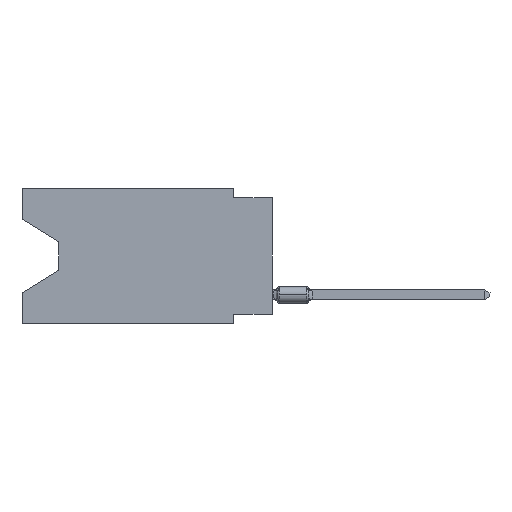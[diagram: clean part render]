
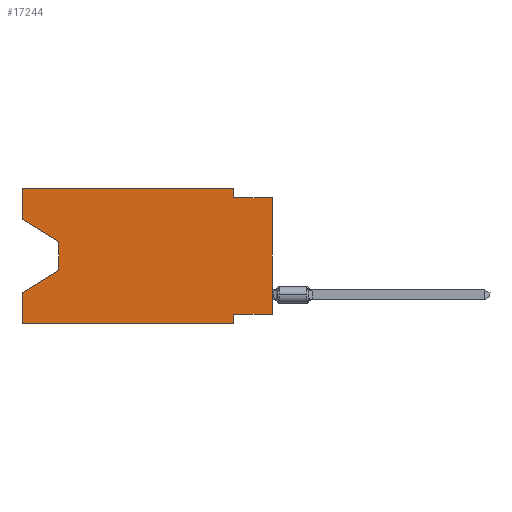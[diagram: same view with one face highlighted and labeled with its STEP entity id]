
A CAD part, left-side view. The second image highlights one B-rep face of the part: STEP entity #17244.
In plain terms, the highlighted planar face has unit normal (-1, 0, 0).
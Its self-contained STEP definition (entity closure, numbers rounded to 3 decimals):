
#54 = VECTOR ( 'NONE', #8513, 1000. ) ;
#129 = VERTEX_POINT ( 'NONE', #4464 ) ;
#520 = DIRECTION ( 'NONE',  ( 0., 0., 1. ) ) ;
#578 = CARTESIAN_POINT ( 'NONE',  ( 0., 2.54, 0. ) ) ;
#824 = CARTESIAN_POINT ( 'NONE',  ( 0., 2.54, -8.89 ) ) ;
#1201 = ORIENTED_EDGE ( 'NONE', *, *, #9714, .F. ) ;
#1211 = CARTESIAN_POINT ( 'NONE',  ( 0., 13.97, -5.385 ) ) ;
#1438 = CARTESIAN_POINT ( 'NONE',  ( 0., 16.383, -8.89 ) ) ;
#1601 = VECTOR ( 'NONE', #7014, 1000. ) ;
#1841 = EDGE_CURVE ( 'NONE', #129, #2615, #18291, .T. ) ;
#1871 = VECTOR ( 'NONE', #10089, 1000. ) ;
#1890 = VECTOR ( 'NONE', #2904, 1000. ) ;
#1977 = CARTESIAN_POINT ( 'NONE',  ( 0., 16.383, 0. ) ) ;
#2011 = LINE ( 'NONE', #16816, #14824 ) ;
#2221 = ORIENTED_EDGE ( 'NONE', *, *, #5392, .F. ) ;
#2327 = LINE ( 'NONE', #15957, #54 ) ;
#2352 = LINE ( 'NONE', #11203, #17663 ) ;
#2615 = VERTEX_POINT ( 'NONE', #17131 ) ;
#2904 = DIRECTION ( 'NONE',  ( 0., 0., -1. ) ) ;
#2983 = EDGE_CURVE ( 'NONE', #18612, #15103, #2011, .T. ) ;
#3115 = DIRECTION ( 'NONE',  ( 0., -1., 0. ) ) ;
#3797 = CARTESIAN_POINT ( 'NONE',  ( 0., 16.383, -6.852 ) ) ;
#3887 = EDGE_CURVE ( 'NONE', #11784, #18872, #2352, .T. ) ;
#3984 = CARTESIAN_POINT ( 'NONE',  ( 0., 16.383, -8.89 ) ) ;
#4029 = VECTOR ( 'NONE', #14144, 1000. ) ;
#4115 = CARTESIAN_POINT ( 'NONE',  ( 0., 0., -8.255 ) ) ;
#4148 = ORIENTED_EDGE ( 'NONE', *, *, #18192, .T. ) ;
#4203 = ORIENTED_EDGE ( 'NONE', *, *, #16361, .F. ) ;
#4351 = LINE ( 'NONE', #19168, #1601 ) ;
#4464 = CARTESIAN_POINT ( 'NONE',  ( 0., 0., -8.255 ) ) ;
#4710 = EDGE_CURVE ( 'NONE', #11416, #5020, #19303, .T. ) ;
#5020 = VERTEX_POINT ( 'NONE', #824 ) ;
#5133 = DIRECTION ( 'NONE',  ( 0., -1., 0. ) ) ;
#5187 = ORIENTED_EDGE ( 'NONE', *, *, #1841, .T. ) ;
#5279 = CARTESIAN_POINT ( 'NONE',  ( 0., 16.383, 0. ) ) ;
#5392 = EDGE_CURVE ( 'NONE', #15103, #12146, #8086, .T. ) ;
#5460 = VECTOR ( 'NONE', #10400, 1000. ) ;
#5760 = ORIENTED_EDGE ( 'NONE', *, *, #18810, .F. ) ;
#6325 = VECTOR ( 'NONE', #520, 1000. ) ;
#6357 = LINE ( 'NONE', #16739, #10652 ) ;
#6530 = DIRECTION ( 'NONE',  ( 0., 0., 1. ) ) ;
#6600 = VECTOR ( 'NONE', #5133, 1000. ) ;
#6723 = ORIENTED_EDGE ( 'NONE', *, *, #10251, .F. ) ;
#7014 = DIRECTION ( 'NONE',  ( 0., -0.855, -0.519 ) ) ;
#7044 = LINE ( 'NONE', #11666, #1871 ) ;
#7783 = ORIENTED_EDGE ( 'NONE', *, *, #4710, .T. ) ;
#8004 = CARTESIAN_POINT ( 'NONE',  ( 0., 0., 0. ) ) ;
#8086 = LINE ( 'NONE', #18577, #6600 ) ;
#8252 = ORIENTED_EDGE ( 'NONE', *, *, #9844, .F. ) ;
#8343 = DIRECTION ( 'NONE',  ( 0., 0.855, -0.519 ) ) ;
#8513 = DIRECTION ( 'NONE',  ( 0., 0., -1. ) ) ;
#9409 = AXIS2_PLACEMENT_3D ( 'NONE', #5279, #12660, #9807 ) ;
#9714 = EDGE_CURVE ( 'NONE', #12146, #14442, #12380, .T. ) ;
#9807 = DIRECTION ( 'NONE',  ( 0., 0., -1. ) ) ;
#9836 = ORIENTED_EDGE ( 'NONE', *, *, #3887, .T. ) ;
#9844 = EDGE_CURVE ( 'NONE', #129, #14368, #9909, .T. ) ;
#9909 = LINE ( 'NONE', #4115, #16266 ) ;
#10089 = DIRECTION ( 'NONE',  ( 0., 0., 1. ) ) ;
#10251 = EDGE_CURVE ( 'NONE', #11416, #18872, #7044, .T. ) ;
#10400 = DIRECTION ( 'NONE',  ( 0., -1., 0. ) ) ;
#10652 = VECTOR ( 'NONE', #3115, 1000. ) ;
#10653 = CARTESIAN_POINT ( 'NONE',  ( 0., 2.54, -0.635 ) ) ;
#11107 = FACE_OUTER_BOUND ( 'NONE', #19220, .T. ) ;
#11203 = CARTESIAN_POINT ( 'NONE',  ( 0., 13.97, -5.385 ) ) ;
#11416 = VERTEX_POINT ( 'NONE', #3984 ) ;
#11666 = CARTESIAN_POINT ( 'NONE',  ( 0., 16.383, 0. ) ) ;
#11784 = VERTEX_POINT ( 'NONE', #1211 ) ;
#12146 = VERTEX_POINT ( 'NONE', #15216 ) ;
#12380 = LINE ( 'NONE', #578, #4029 ) ;
#12660 = DIRECTION ( 'NONE',  ( 1., 0., 0. ) ) ;
#13013 = CARTESIAN_POINT ( 'NONE',  ( 0., 13.97, -3.505 ) ) ;
#14011 = CARTESIAN_POINT ( 'NONE',  ( 0., 16.383, -2.038 ) ) ;
#14144 = DIRECTION ( 'NONE',  ( 0., 0., -1. ) ) ;
#14368 = VERTEX_POINT ( 'NONE', #17599 ) ;
#14417 = PLANE ( 'NONE',  #9409 ) ;
#14442 = VERTEX_POINT ( 'NONE', #10653 ) ;
#14677 = LINE ( 'NONE', #13013, #1890 ) ;
#14824 = VECTOR ( 'NONE', #6530, 1000. ) ;
#15103 = VERTEX_POINT ( 'NONE', #1977 ) ;
#15216 = CARTESIAN_POINT ( 'NONE',  ( 0., 2.54, 0. ) ) ;
#15331 = VERTEX_POINT ( 'NONE', #18239 ) ;
#15410 = ORIENTED_EDGE ( 'NONE', *, *, #2983, .F. ) ;
#15694 = ORIENTED_EDGE ( 'NONE', *, *, #17860, .T. ) ;
#15877 = DIRECTION ( 'NONE',  ( 0., 1., 0. ) ) ;
#15957 = CARTESIAN_POINT ( 'NONE',  ( 0., 2.54, -8.89 ) ) ;
#16266 = VECTOR ( 'NONE', #15877, 1000. ) ;
#16361 = EDGE_CURVE ( 'NONE', #14442, #2615, #6357, .T. ) ;
#16739 = CARTESIAN_POINT ( 'NONE',  ( 0., 0., -0.635 ) ) ;
#16816 = CARTESIAN_POINT ( 'NONE',  ( 0., 16.383, 0. ) ) ;
#17131 = CARTESIAN_POINT ( 'NONE',  ( 0., 0., -0.635 ) ) ;
#17244 = ADVANCED_FACE ( 'NONE', ( #11107 ), #14417, .F. ) ;
#17599 = CARTESIAN_POINT ( 'NONE',  ( 0., 2.54, -8.255 ) ) ;
#17663 = VECTOR ( 'NONE', #8343, 1000. ) ;
#17860 = EDGE_CURVE ( 'NONE', #15331, #11784, #14677, .T. ) ;
#18192 = EDGE_CURVE ( 'NONE', #18612, #15331, #4351, .T. ) ;
#18239 = CARTESIAN_POINT ( 'NONE',  ( 0., 13.97, -3.505 ) ) ;
#18291 = LINE ( 'NONE', #8004, #6325 ) ;
#18577 = CARTESIAN_POINT ( 'NONE',  ( 0., 16.383, 0. ) ) ;
#18612 = VERTEX_POINT ( 'NONE', #14011 ) ;
#18810 = EDGE_CURVE ( 'NONE', #14368, #5020, #2327, .T. ) ;
#18872 = VERTEX_POINT ( 'NONE', #3797 ) ;
#19168 = CARTESIAN_POINT ( 'NONE',  ( 0., 16.383, -2.038 ) ) ;
#19220 = EDGE_LOOP ( 'NONE', ( #4148, #15694, #9836, #6723, #7783, #5760, #8252, #5187, #4203, #1201, #2221, #15410 ) ) ;
#19303 = LINE ( 'NONE', #1438, #5460 ) ;
